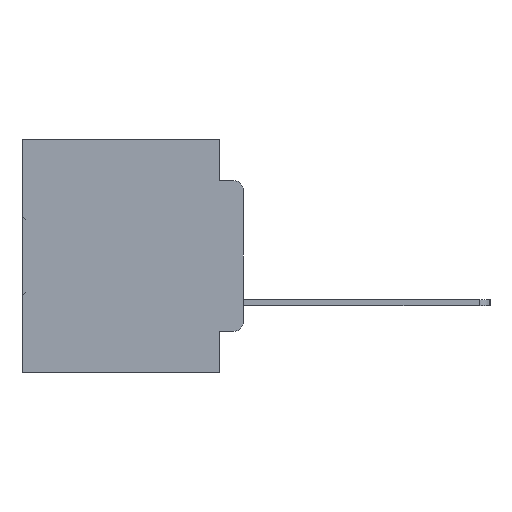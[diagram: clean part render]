
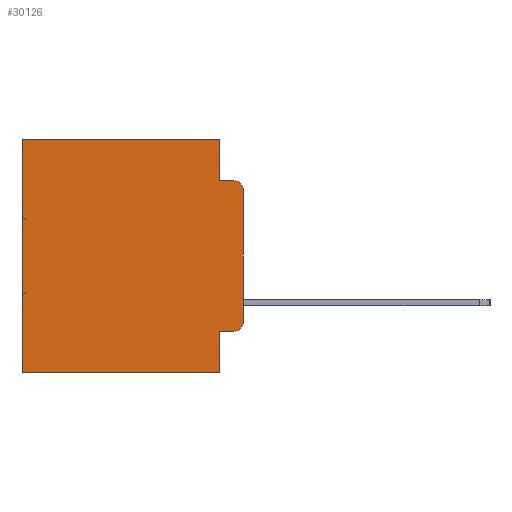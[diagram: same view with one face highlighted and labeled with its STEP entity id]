
A CAD part, left-side view. The second image highlights one B-rep face of the part: STEP entity #30126.
In plain terms, the highlighted planar face has unit normal (-1, 0, 0).
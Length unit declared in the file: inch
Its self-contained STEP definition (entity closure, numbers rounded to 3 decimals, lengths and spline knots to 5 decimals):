
#647 = CARTESIAN_POINT ( 'NONE',  ( 0.298, 0.051, -0.4115 ) ) ;
#867 = VECTOR ( 'NONE', #17312, 39.37008 ) ;
#876 = VECTOR ( 'NONE', #30607, 39.37008 ) ;
#1067 = CARTESIAN_POINT ( 'NONE',  ( 0.298, 0., -0.5 ) ) ;
#1069 = VECTOR ( 'NONE', #34402, 39.37008 ) ;
#1773 = LINE ( 'NONE', #1067, #876 ) ;
#1816 = VERTEX_POINT ( 'NONE', #30818 ) ;
#1962 = LINE ( 'NONE', #31862, #1069 ) ;
#2032 = VECTOR ( 'NONE', #17096, 39.37008 ) ;
#2135 = VERTEX_POINT ( 'NONE', #34330 ) ;
#2290 = LINE ( 'NONE', #12589, #8754 ) ;
#2823 = CARTESIAN_POINT ( 'NONE',  ( 0.298, 0.473, 0. ) ) ;
#2894 = LINE ( 'NONE', #647, #2032 ) ;
#2970 = VERTEX_POINT ( 'NONE', #8602 ) ;
#3643 = DIRECTION ( 'NONE',  ( 1., 0., 0. ) ) ;
#3940 = ORIENTED_EDGE ( 'NONE', *, *, #21591, .F. ) ;
#5022 = AXIS2_PLACEMENT_3D ( 'NONE', #9148, #27873, #11881 ) ;
#5217 = CARTESIAN_POINT ( 'NONE',  ( 0.298, 0., 0. ) ) ;
#5854 = EDGE_CURVE ( 'NONE', #19211, #1816, #2290, .T. ) ;
#7010 = CARTESIAN_POINT ( 'NONE',  ( 0.298, 0.051, -0.5 ) ) ;
#8602 = CARTESIAN_POINT ( 'NONE',  ( 0.298, 0., -0.3915 ) ) ;
#8754 = VECTOR ( 'NONE', #18082, 39.37008 ) ;
#9000 = VECTOR ( 'NONE', #33960, 39.37008 ) ;
#9108 = ORIENTED_EDGE ( 'NONE', *, *, #30886, .F. ) ;
#9148 = CARTESIAN_POINT ( 'NONE',  ( 0.298, 0.02, -0.1085 ) ) ;
#9445 = LINE ( 'NONE', #5217, #23031 ) ;
#9463 = EDGE_CURVE ( 'NONE', #10804, #2135, #2894, .T. ) ;
#9588 = ORIENTED_EDGE ( 'NONE', *, *, #13861, .F. ) ;
#10138 = AXIS2_PLACEMENT_3D ( 'NONE', #28612, #12649, #31207 ) ;
#10804 = VERTEX_POINT ( 'NONE', #31068 ) ;
#11016 = EDGE_CURVE ( 'NONE', #21083, #27763, #1962, .T. ) ;
#11822 = CARTESIAN_POINT ( 'NONE',  ( 0.298, 0.051, 0. ) ) ;
#11881 = DIRECTION ( 'NONE',  ( 0., 0., -1. ) ) ;
#12385 = LINE ( 'NONE', #16305, #25039 ) ;
#12589 = CARTESIAN_POINT ( 'NONE',  ( 0.298, 0.051, -0.0885 ) ) ;
#12649 = DIRECTION ( 'NONE',  ( -1., 0., 0. ) ) ;
#13188 = EDGE_CURVE ( 'NONE', #21083, #19211, #17201, .T. ) ;
#13861 = EDGE_CURVE ( 'NONE', #18985, #31482, #1773, .T. ) ;
#16271 = LINE ( 'NONE', #31412, #9000 ) ;
#16305 = CARTESIAN_POINT ( 'NONE',  ( 0.298, 0.473, 0. ) ) ;
#16841 = CARTESIAN_POINT ( 'NONE',  ( 0.298, 0., -0.1085 ) ) ;
#17096 = DIRECTION ( 'NONE',  ( 0., -1., 0. ) ) ;
#17201 = LINE ( 'NONE', #11822, #867 ) ;
#17312 = DIRECTION ( 'NONE',  ( 0., 0., -1. ) ) ;
#18082 = DIRECTION ( 'NONE',  ( 0., -1., 0. ) ) ;
#18964 = CARTESIAN_POINT ( 'NONE',  ( 0.298, 0.051, -0.0885 ) ) ;
#18985 = VERTEX_POINT ( 'NONE', #7010 ) ;
#19053 = DIRECTION ( 'NONE',  ( 0., 0., -1. ) ) ;
#19156 = ORIENTED_EDGE ( 'NONE', *, *, #30284, .T. ) ;
#19211 = VERTEX_POINT ( 'NONE', #18964 ) ;
#19295 = FACE_OUTER_BOUND ( 'NONE', #24035, .T. ) ;
#19964 = VERTEX_POINT ( 'NONE', #16841 ) ;
#20011 = CARTESIAN_POINT ( 'NONE',  ( 0.298, 0., 0. ) ) ;
#20637 = ORIENTED_EDGE ( 'NONE', *, *, #22233, .T. ) ;
#21083 = VERTEX_POINT ( 'NONE', #26742 ) ;
#21393 = CIRCLE ( 'NONE', #10138, 0.02 ) ;
#21591 = EDGE_CURVE ( 'NONE', #19964, #2970, #9445, .T. ) ;
#22233 = EDGE_CURVE ( 'NONE', #27763, #31482, #12385, .T. ) ;
#22726 = DIRECTION ( 'NONE',  ( 0., 0., -1. ) ) ;
#23031 = VECTOR ( 'NONE', #24241, 39.37008 ) ;
#23065 = ORIENTED_EDGE ( 'NONE', *, *, #11016, .T. ) ;
#24035 = EDGE_LOOP ( 'NONE', ( #3940, #27685, #30405, #34611, #23065, #20637, #9588, #9108, #27452, #19156 ) ) ;
#24241 = DIRECTION ( 'NONE',  ( 0., 0., -1. ) ) ;
#24589 = CIRCLE ( 'NONE', #5022, 0.02 ) ;
#25039 = VECTOR ( 'NONE', #19053, 39.37008 ) ;
#26742 = CARTESIAN_POINT ( 'NONE',  ( 0.298, 0.051, 0. ) ) ;
#27452 = ORIENTED_EDGE ( 'NONE', *, *, #9463, .T. ) ;
#27685 = ORIENTED_EDGE ( 'NONE', *, *, #28577, .T. ) ;
#27688 = PLANE ( 'NONE',  #30422 ) ;
#27763 = VERTEX_POINT ( 'NONE', #2823 ) ;
#27873 = DIRECTION ( 'NONE',  ( -1., 0., 0. ) ) ;
#28577 = EDGE_CURVE ( 'NONE', #19964, #1816, #24589, .T. ) ;
#28612 = CARTESIAN_POINT ( 'NONE',  ( 0.298, 0.02, -0.3915 ) ) ;
#30126 = ADVANCED_FACE ( 'NONE', ( #19295 ), #27688, .F. ) ;
#30284 = EDGE_CURVE ( 'NONE', #2135, #2970, #21393, .T. ) ;
#30405 = ORIENTED_EDGE ( 'NONE', *, *, #5854, .F. ) ;
#30422 = AXIS2_PLACEMENT_3D ( 'NONE', #20011, #3643, #22726 ) ;
#30607 = DIRECTION ( 'NONE',  ( 0., 1., 0. ) ) ;
#30818 = CARTESIAN_POINT ( 'NONE',  ( 0.298, 0.02, -0.0885 ) ) ;
#30886 = EDGE_CURVE ( 'NONE', #10804, #18985, #16271, .T. ) ;
#31068 = CARTESIAN_POINT ( 'NONE',  ( 0.298, 0.051, -0.4115 ) ) ;
#31207 = DIRECTION ( 'NONE',  ( 0., 0., -1. ) ) ;
#31412 = CARTESIAN_POINT ( 'NONE',  ( 0.298, 0.051, 0. ) ) ;
#31482 = VERTEX_POINT ( 'NONE', #33808 ) ;
#31862 = CARTESIAN_POINT ( 'NONE',  ( 0.298, 0., 0. ) ) ;
#33808 = CARTESIAN_POINT ( 'NONE',  ( 0.298, 0.473, -0.5 ) ) ;
#33960 = DIRECTION ( 'NONE',  ( 0., 0., -1. ) ) ;
#34330 = CARTESIAN_POINT ( 'NONE',  ( 0.298, 0.02, -0.4115 ) ) ;
#34402 = DIRECTION ( 'NONE',  ( 0., 1., 0. ) ) ;
#34611 = ORIENTED_EDGE ( 'NONE', *, *, #13188, .F. ) ;
